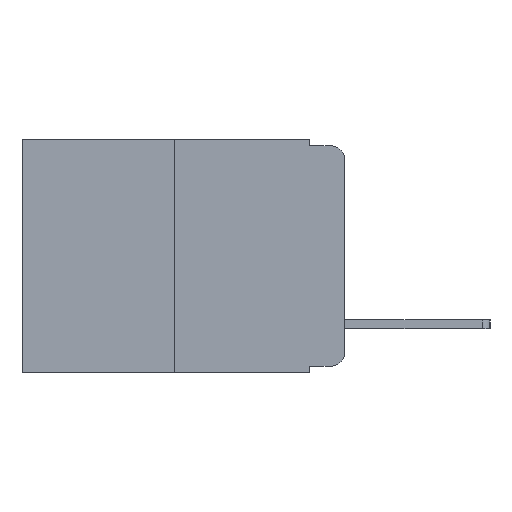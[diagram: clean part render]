
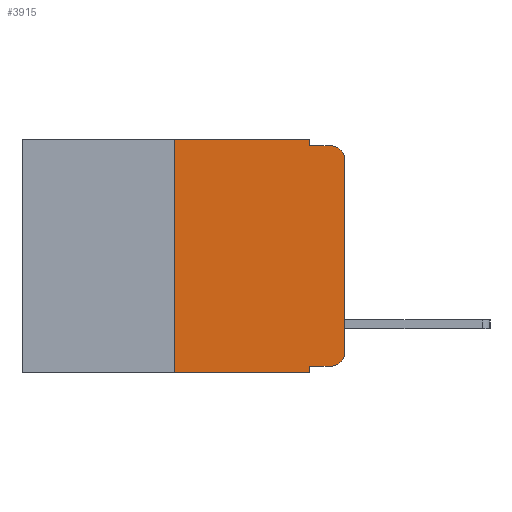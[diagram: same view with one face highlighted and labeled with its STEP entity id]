
A CAD part, left-side view. The second image highlights one B-rep face of the part: STEP entity #3915.
In plain terms, the highlighted planar face has unit normal (-1, 0, 0).
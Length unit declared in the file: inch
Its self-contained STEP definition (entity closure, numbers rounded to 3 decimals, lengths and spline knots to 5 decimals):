
#20 = EDGE_CURVE ( 'NONE', #142, #9226, #5378, .T. ) ;
#59 = LINE ( 'NONE', #8482, #9393 ) ;
#142 = VERTEX_POINT ( 'NONE', #11309 ) ;
#145 = FACE_OUTER_BOUND ( 'NONE', #7760, .T. ) ;
#252 = AXIS2_PLACEMENT_3D ( 'NONE', #5621, #10364, #8969 ) ;
#564 = LINE ( 'NONE', #6323, #7266 ) ;
#673 = VERTEX_POINT ( 'NONE', #2611 ) ;
#1024 = DIRECTION ( 'NONE',  ( -1., 0., 0. ) ) ;
#1503 = VERTEX_POINT ( 'NONE', #9457 ) ;
#1652 = CARTESIAN_POINT ( 'NONE',  ( 0., 0.25, 0. ) ) ;
#2207 = CARTESIAN_POINT ( 'NONE',  ( 0., 0.051, -0.01 ) ) ;
#2547 = CIRCLE ( 'NONE', #9148, 0.02 ) ;
#2550 = DIRECTION ( 'NONE',  ( 0., 0., 1. ) ) ;
#2611 = CARTESIAN_POINT ( 'NONE',  ( 0., 0.051, -0.343 ) ) ;
#2891 = VERTEX_POINT ( 'NONE', #3871 ) ;
#3298 = CARTESIAN_POINT ( 'NONE',  ( 0., 0.051, 0. ) ) ;
#3363 = VERTEX_POINT ( 'NONE', #6470 ) ;
#3408 = ORIENTED_EDGE ( 'NONE', *, *, #10133, .T. ) ;
#3443 = VECTOR ( 'NONE', #4184, 39.37008 ) ;
#3471 = CARTESIAN_POINT ( 'NONE',  ( 0., 0.473, -0.343 ) ) ;
#3846 = VERTEX_POINT ( 'NONE', #7617 ) ;
#3871 = CARTESIAN_POINT ( 'NONE',  ( 0., 0.25, 0. ) ) ;
#3885 = CARTESIAN_POINT ( 'NONE',  ( 0., 0.02, -0.313 ) ) ;
#3915 = ADVANCED_FACE ( 'NONE', ( #145 ), #8218, .F. ) ;
#3923 = DIRECTION ( 'NONE',  ( -1., 0., 0. ) ) ;
#3924 = ORIENTED_EDGE ( 'NONE', *, *, #10190, .T. ) ;
#3972 = CARTESIAN_POINT ( 'NONE',  ( 0., 0.051, -0.333 ) ) ;
#4076 = DIRECTION ( 'NONE',  ( 0., -1., 0. ) ) ;
#4143 = ORIENTED_EDGE ( 'NONE', *, *, #10398, .F. ) ;
#4184 = DIRECTION ( 'NONE',  ( 0., 0., -1. ) ) ;
#4568 = CARTESIAN_POINT ( 'NONE',  ( 0., 0.051, -0.01 ) ) ;
#4757 = ORIENTED_EDGE ( 'NONE', *, *, #10460, .F. ) ;
#4891 = ORIENTED_EDGE ( 'NONE', *, *, #9427, .F. ) ;
#4963 = ORIENTED_EDGE ( 'NONE', *, *, #10614, .F. ) ;
#5017 = ORIENTED_EDGE ( 'NONE', *, *, #7994, .T. ) ;
#5161 = ORIENTED_EDGE ( 'NONE', *, *, #10685, .F. ) ;
#5293 = ORIENTED_EDGE ( 'NONE', *, *, #10808, .T. ) ;
#5342 = DIRECTION ( 'NONE',  ( 0., 0., -1. ) ) ;
#5378 = CIRCLE ( 'NONE', #9535, 0.02 ) ;
#5431 = ORIENTED_EDGE ( 'NONE', *, *, #20, .T. ) ;
#5610 = LINE ( 'NONE', #7951, #7668 ) ;
#5621 = CARTESIAN_POINT ( 'NONE',  ( 0., 0.473, 0. ) ) ;
#6267 = DIRECTION ( 'NONE',  ( 0., -1., 0. ) ) ;
#6323 = CARTESIAN_POINT ( 'NONE',  ( 0., 0., 0. ) ) ;
#6339 = LINE ( 'NONE', #3471, #10505 ) ;
#6432 = CARTESIAN_POINT ( 'NONE',  ( 0., 0.02, -0.03 ) ) ;
#6470 = CARTESIAN_POINT ( 'NONE',  ( 0., 0.051, 0. ) ) ;
#6698 = LINE ( 'NONE', #1652, #8488 ) ;
#6773 = VERTEX_POINT ( 'NONE', #9403 ) ;
#6865 = VECTOR ( 'NONE', #4076, 39.37008 ) ;
#7111 = LINE ( 'NONE', #7159, #11194 ) ;
#7119 = LINE ( 'NONE', #2207, #6865 ) ;
#7159 = CARTESIAN_POINT ( 'NONE',  ( 0., 0.051, -0.333 ) ) ;
#7266 = VECTOR ( 'NONE', #11267, 39.37008 ) ;
#7320 = DIRECTION ( 'NONE',  ( 0., 0., -1. ) ) ;
#7617 = CARTESIAN_POINT ( 'NONE',  ( 0., 0.25, -0.343 ) ) ;
#7668 = VECTOR ( 'NONE', #9597, 39.37008 ) ;
#7760 = EDGE_LOOP ( 'NONE', ( #3408, #3924, #4143, #4757, #4891, #4963, #5017, #5161, #5293, #5431 ) ) ;
#7951 = CARTESIAN_POINT ( 'NONE',  ( 0., 0.051, 0. ) ) ;
#7994 = EDGE_CURVE ( 'NONE', #3846, #673, #6339, .T. ) ;
#8112 = LINE ( 'NONE', #3298, #3443 ) ;
#8218 = PLANE ( 'NONE',  #252 ) ;
#8482 = CARTESIAN_POINT ( 'NONE',  ( 0., 0.473, 0. ) ) ;
#8488 = VECTOR ( 'NONE', #2550, 39.37008 ) ;
#8969 = DIRECTION ( 'NONE',  ( 0., 0., -1. ) ) ;
#9081 = CARTESIAN_POINT ( 'NONE',  ( 0., 0., -0.313 ) ) ;
#9148 = AXIS2_PLACEMENT_3D ( 'NONE', #6432, #1024, #7320 ) ;
#9226 = VERTEX_POINT ( 'NONE', #9081 ) ;
#9285 = DIRECTION ( 'NONE',  ( 0., -1., 0. ) ) ;
#9393 = VECTOR ( 'NONE', #9285, 39.37008 ) ;
#9403 = CARTESIAN_POINT ( 'NONE',  ( 0., 0.02, -0.01 ) ) ;
#9427 = EDGE_CURVE ( 'NONE', #2891, #3363, #59, .T. ) ;
#9457 = CARTESIAN_POINT ( 'NONE',  ( 0., 0., -0.03 ) ) ;
#9535 = AXIS2_PLACEMENT_3D ( 'NONE', #3885, #3923, #5342 ) ;
#9597 = DIRECTION ( 'NONE',  ( 0., 0., -1. ) ) ;
#10133 = EDGE_CURVE ( 'NONE', #9226, #1503, #564, .T. ) ;
#10190 = EDGE_CURVE ( 'NONE', #1503, #6773, #2547, .T. ) ;
#10364 = DIRECTION ( 'NONE',  ( 1., 0., 0. ) ) ;
#10398 = EDGE_CURVE ( 'NONE', #10890, #6773, #7119, .T. ) ;
#10460 = EDGE_CURVE ( 'NONE', #3363, #10890, #8112, .T. ) ;
#10505 = VECTOR ( 'NONE', #11069, 39.37008 ) ;
#10614 = EDGE_CURVE ( 'NONE', #3846, #2891, #6698, .T. ) ;
#10685 = EDGE_CURVE ( 'NONE', #11199, #673, #5610, .T. ) ;
#10808 = EDGE_CURVE ( 'NONE', #11199, #142, #7111, .T. ) ;
#10890 = VERTEX_POINT ( 'NONE', #4568 ) ;
#11069 = DIRECTION ( 'NONE',  ( 0., -1., 0. ) ) ;
#11194 = VECTOR ( 'NONE', #6267, 39.37008 ) ;
#11199 = VERTEX_POINT ( 'NONE', #3972 ) ;
#11267 = DIRECTION ( 'NONE',  ( 0., 0., 1. ) ) ;
#11309 = CARTESIAN_POINT ( 'NONE',  ( 0., 0.02, -0.333 ) ) ;
